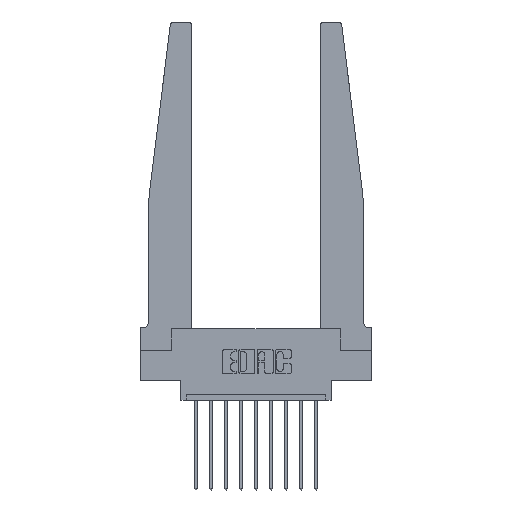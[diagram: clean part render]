
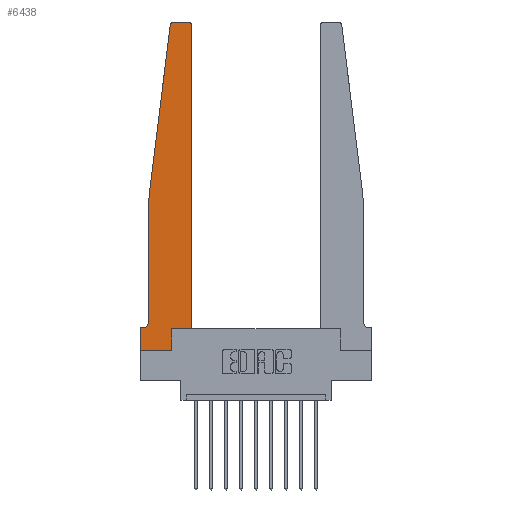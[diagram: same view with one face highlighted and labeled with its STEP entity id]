
A CAD part, top view. The second image highlights one B-rep face of the part: STEP entity #6438.
In plain terms, the highlighted planar face has unit normal (0, 0, 1).
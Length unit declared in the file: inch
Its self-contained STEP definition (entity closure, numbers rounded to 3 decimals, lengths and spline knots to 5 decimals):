
#62 = ORIENTED_EDGE ( 'NONE', *, *, #8551, .T. ) ;
#111 = VECTOR ( 'NONE', #5114, 39.37008 ) ;
#155 = DIRECTION ( 'NONE',  ( 1., 0., 0. ) ) ;
#187 = VECTOR ( 'NONE', #10108, 39.37008 ) ;
#193 = VERTEX_POINT ( 'NONE', #6606 ) ;
#394 = EDGE_CURVE ( 'NONE', #11212, #14077, #14646, .T. ) ;
#642 = CARTESIAN_POINT ( 'NONE',  ( 0., 0.1875, 0.37 ) ) ;
#925 = LINE ( 'NONE', #1079, #187 ) ;
#930 = DIRECTION ( 'NONE',  ( -0.122, -0.992, 0. ) ) ;
#1079 = CARTESIAN_POINT ( 'NONE',  ( 0., 0., 0.37 ) ) ;
#1277 = VECTOR ( 'NONE', #10256, 39.37008 ) ;
#1370 = DIRECTION ( 'NONE',  ( -1., 0., 0. ) ) ;
#1457 = CARTESIAN_POINT ( 'NONE',  ( 0.065, 0.1875, 0.37 ) ) ;
#1502 = LINE ( 'NONE', #12914, #9621 ) ;
#1554 = CIRCLE ( 'NONE', #9604, 0.05 ) ;
#1585 = CIRCLE ( 'NONE', #11400, 0.03 ) ;
#1609 = DIRECTION ( 'NONE',  ( 1., 0., 0. ) ) ;
#1798 = DIRECTION ( 'NONE',  ( 0., -1., 0. ) ) ;
#1815 = VERTEX_POINT ( 'NONE', #13273 ) ;
#1843 = LINE ( 'NONE', #1457, #12615 ) ;
#1890 = ORIENTED_EDGE ( 'NONE', *, *, #14453, .T. ) ;
#1974 = CARTESIAN_POINT ( 'NONE',  ( 0.015, 0.2375, 0.37 ) ) ;
#1979 = EDGE_CURVE ( 'NONE', #5306, #1815, #10615, .T. ) ;
#2158 = CARTESIAN_POINT ( 'NONE',  ( 0.425, 0.18, 0.37 ) ) ;
#2364 = ORIENTED_EDGE ( 'NONE', *, *, #6770, .T. ) ;
#2723 = LINE ( 'NONE', #6619, #14601 ) ;
#2869 = VERTEX_POINT ( 'NONE', #14921 ) ;
#2924 = ORIENTED_EDGE ( 'NONE', *, *, #394, .T. ) ;
#3075 = EDGE_CURVE ( 'NONE', #14080, #11212, #1585, .T. ) ;
#3347 = CARTESIAN_POINT ( 'NONE',  ( 0.27653, 2.75, 0.37 ) ) ;
#3646 = CARTESIAN_POINT ( 'NONE',  ( 0.2605, 0., 0.37 ) ) ;
#3773 = LINE ( 'NONE', #8783, #13460 ) ;
#3821 = EDGE_CURVE ( 'NONE', #2869, #13388, #1554, .T. ) ;
#4105 = VERTEX_POINT ( 'NONE', #7919 ) ;
#4110 = CARTESIAN_POINT ( 'NONE',  ( 0.015, 0.1875, 0.37 ) ) ;
#4485 = CARTESIAN_POINT ( 'NONE',  ( 0.065, 1.25, 0.37 ) ) ;
#4533 = CARTESIAN_POINT ( 'NONE',  ( 0.425, 0.18, 0.37 ) ) ;
#5079 = LINE ( 'NONE', #9352, #8484 ) ;
#5114 = DIRECTION ( 'NONE',  ( 0., -1., 0. ) ) ;
#5306 = VERTEX_POINT ( 'NONE', #4533 ) ;
#5476 = CARTESIAN_POINT ( 'NONE',  ( 0.395, 2.75, 0.37 ) ) ;
#5930 = VERTEX_POINT ( 'NONE', #5476 ) ;
#5985 = DIRECTION ( 'NONE',  ( 0., 0., 1. ) ) ;
#6012 = PLANE ( 'NONE',  #9907 ) ;
#6217 = CARTESIAN_POINT ( 'NONE',  ( 0.065, 1.25, 0.37 ) ) ;
#6418 = CARTESIAN_POINT ( 'NONE',  ( 0.27653, 2.72, 0.37 ) ) ;
#6438 = ADVANCED_FACE ( 'NONE', ( #14247 ), #6012, .T. ) ;
#6471 = DIRECTION ( 'NONE',  ( 0., 0., 1. ) ) ;
#6606 = CARTESIAN_POINT ( 'NONE',  ( 0.2605, 0.18, 0.37 ) ) ;
#6619 = CARTESIAN_POINT ( 'NONE',  ( 0., 0., 0.37 ) ) ;
#6770 = EDGE_CURVE ( 'NONE', #14529, #8045, #925, .T. ) ;
#7020 = LINE ( 'NONE', #6217, #111 ) ;
#7356 = ORIENTED_EDGE ( 'NONE', *, *, #3821, .T. ) ;
#7647 = VECTOR ( 'NONE', #930, 39.37008 ) ;
#7751 = DIRECTION ( 'NONE',  ( -1., 0., 0. ) ) ;
#7919 = CARTESIAN_POINT ( 'NONE',  ( 0., 0.1875, 0.37 ) ) ;
#8045 = VERTEX_POINT ( 'NONE', #3646 ) ;
#8375 = ORIENTED_EDGE ( 'NONE', *, *, #3075, .T. ) ;
#8484 = VECTOR ( 'NONE', #13832, 39.37008 ) ;
#8551 = EDGE_CURVE ( 'NONE', #193, #5306, #5079, .T. ) ;
#8555 = EDGE_LOOP ( 'NONE', ( #11835, #8375, #2924, #1890, #7356, #13287, #13324, #2364, #8686, #62, #13088, #12209 ) ) ;
#8686 = ORIENTED_EDGE ( 'NONE', *, *, #10848, .T. ) ;
#8758 = DIRECTION ( 'NONE',  ( 1., 0., 0. ) ) ;
#8783 = CARTESIAN_POINT ( 'NONE',  ( 0.25, 2.75, 0.37 ) ) ;
#9352 = CARTESIAN_POINT ( 'NONE',  ( 0.425, 0.18, 0.37 ) ) ;
#9376 = EDGE_CURVE ( 'NONE', #5930, #14080, #3773, .T. ) ;
#9445 = DIRECTION ( 'NONE',  ( 0., 1., 0. ) ) ;
#9604 = AXIS2_PLACEMENT_3D ( 'NONE', #1974, #12277, #7751 ) ;
#9621 = VECTOR ( 'NONE', #9445, 39.37008 ) ;
#9907 = AXIS2_PLACEMENT_3D ( 'NONE', #642, #11999, #1609 ) ;
#10009 = CARTESIAN_POINT ( 'NONE',  ( 0., 0., 0.37 ) ) ;
#10108 = DIRECTION ( 'NONE',  ( 1., 0., 0. ) ) ;
#10256 = DIRECTION ( 'NONE',  ( 0., 1., 0. ) ) ;
#10501 = CARTESIAN_POINT ( 'NONE',  ( 0.395, 2.72, 0.37 ) ) ;
#10615 = LINE ( 'NONE', #2158, #1277 ) ;
#10695 = AXIS2_PLACEMENT_3D ( 'NONE', #10501, #5985, #155 ) ;
#10848 = EDGE_CURVE ( 'NONE', #8045, #193, #1502, .T. ) ;
#11011 = DIRECTION ( 'NONE',  ( -1., 0., 0. ) ) ;
#11209 = CIRCLE ( 'NONE', #10695, 0.03 ) ;
#11212 = VERTEX_POINT ( 'NONE', #11458 ) ;
#11400 = AXIS2_PLACEMENT_3D ( 'NONE', #6418, #6471, #8758 ) ;
#11417 = EDGE_CURVE ( 'NONE', #1815, #5930, #11209, .T. ) ;
#11458 = CARTESIAN_POINT ( 'NONE',  ( 0.24675, 2.72367, 0.37 ) ) ;
#11835 = ORIENTED_EDGE ( 'NONE', *, *, #9376, .T. ) ;
#11999 = DIRECTION ( 'NONE',  ( 0., 0., 1. ) ) ;
#12209 = ORIENTED_EDGE ( 'NONE', *, *, #11417, .T. ) ;
#12276 = EDGE_CURVE ( 'NONE', #13388, #4105, #1843, .T. ) ;
#12277 = DIRECTION ( 'NONE',  ( 0., 0., -1. ) ) ;
#12345 = CARTESIAN_POINT ( 'NONE',  ( 0.065, 1.25, 0.37 ) ) ;
#12615 = VECTOR ( 'NONE', #1370, 39.37008 ) ;
#12841 = EDGE_CURVE ( 'NONE', #4105, #14529, #2723, .T. ) ;
#12914 = CARTESIAN_POINT ( 'NONE',  ( 0.2605, 0.18, 0.37 ) ) ;
#13088 = ORIENTED_EDGE ( 'NONE', *, *, #1979, .T. ) ;
#13273 = CARTESIAN_POINT ( 'NONE',  ( 0.425, 2.72, 0.37 ) ) ;
#13287 = ORIENTED_EDGE ( 'NONE', *, *, #12276, .T. ) ;
#13324 = ORIENTED_EDGE ( 'NONE', *, *, #12841, .T. ) ;
#13388 = VERTEX_POINT ( 'NONE', #4110 ) ;
#13460 = VECTOR ( 'NONE', #11011, 39.37008 ) ;
#13832 = DIRECTION ( 'NONE',  ( 1., 0., 0. ) ) ;
#14077 = VERTEX_POINT ( 'NONE', #4485 ) ;
#14080 = VERTEX_POINT ( 'NONE', #3347 ) ;
#14247 = FACE_OUTER_BOUND ( 'NONE', #8555, .T. ) ;
#14453 = EDGE_CURVE ( 'NONE', #14077, #2869, #7020, .T. ) ;
#14529 = VERTEX_POINT ( 'NONE', #10009 ) ;
#14601 = VECTOR ( 'NONE', #1798, 39.37008 ) ;
#14646 = LINE ( 'NONE', #12345, #7647 ) ;
#14921 = CARTESIAN_POINT ( 'NONE',  ( 0.065, 0.2375, 0.37 ) ) ;
